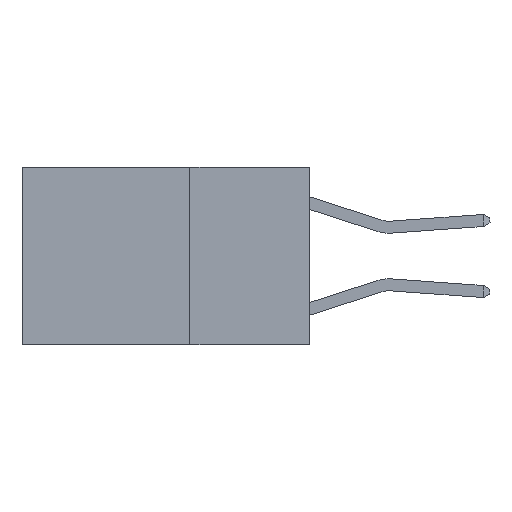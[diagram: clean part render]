
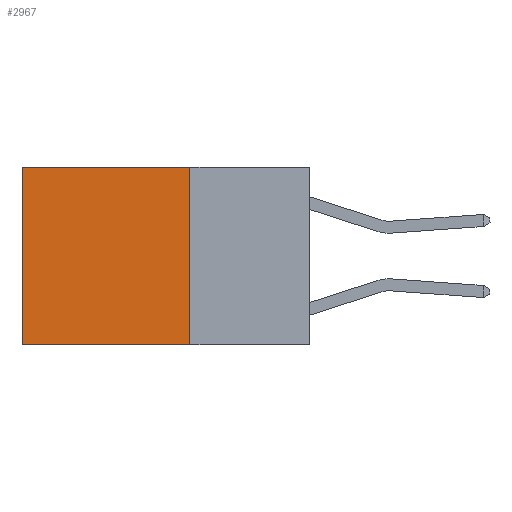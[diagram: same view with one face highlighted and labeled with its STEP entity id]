
A CAD part, left-side view. The second image highlights one B-rep face of the part: STEP entity #2967.
In plain terms, the highlighted planar face has unit normal (-1, 0, 0).
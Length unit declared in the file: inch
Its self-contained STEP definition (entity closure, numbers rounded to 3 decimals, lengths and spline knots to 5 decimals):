
#13 = EDGE_LOOP ( 'NONE', ( #6144, #16299, #10624, #16169 ) ) ;
#386 = DIRECTION ( 'NONE',  ( 0., 0., -1. ) ) ;
#877 = VECTOR ( 'NONE', #18051, 39.37008 ) ;
#1320 = VERTEX_POINT ( 'NONE', #2333 ) ;
#1862 = CARTESIAN_POINT ( 'NONE',  ( 0.2625, 0.6, 0. ) ) ;
#2333 = CARTESIAN_POINT ( 'NONE',  ( 0.2625, 0.6, -0.37 ) ) ;
#2347 = LINE ( 'NONE', #3435, #2872 ) ;
#2629 = PLANE ( 'NONE',  #9972 ) ;
#2872 = VECTOR ( 'NONE', #386, 39.37008 ) ;
#2967 = ADVANCED_FACE ( 'NONE', ( #16172 ), #2629, .F. ) ;
#3435 = CARTESIAN_POINT ( 'NONE',  ( 0.2625, 0.25, 0. ) ) ;
#3938 = CARTESIAN_POINT ( 'NONE',  ( 0.2625, 0.25, 0. ) ) ;
#4616 = CARTESIAN_POINT ( 'NONE',  ( 0.2625, 0.25, 0. ) ) ;
#4956 = EDGE_CURVE ( 'NONE', #8436, #1320, #16092, .T. ) ;
#6003 = LINE ( 'NONE', #15457, #19912 ) ;
#6144 = ORIENTED_EDGE ( 'NONE', *, *, #4956, .T. ) ;
#7473 = CARTESIAN_POINT ( 'NONE',  ( 0.2625, 0.25, -0.37 ) ) ;
#8436 = VERTEX_POINT ( 'NONE', #1862 ) ;
#8684 = DIRECTION ( 'NONE',  ( 0., 1., 0. ) ) ;
#9086 = DIRECTION ( 'NONE',  ( 0., 1., 0. ) ) ;
#9587 = CARTESIAN_POINT ( 'NONE',  ( 0.2625, 0.6, 0. ) ) ;
#9831 = LINE ( 'NONE', #20088, #16014 ) ;
#9972 = AXIS2_PLACEMENT_3D ( 'NONE', #3938, #17127, #12805 ) ;
#10485 = EDGE_CURVE ( 'NONE', #18969, #8436, #6003, .T. ) ;
#10624 = ORIENTED_EDGE ( 'NONE', *, *, #11504, .F. ) ;
#11504 = EDGE_CURVE ( 'NONE', #18969, #17571, #2347, .T. ) ;
#12805 = DIRECTION ( 'NONE',  ( 0., 0., -1. ) ) ;
#15457 = CARTESIAN_POINT ( 'NONE',  ( 0.2625, 0.25, 0. ) ) ;
#16014 = VECTOR ( 'NONE', #8684, 39.37008 ) ;
#16092 = LINE ( 'NONE', #9587, #877 ) ;
#16169 = ORIENTED_EDGE ( 'NONE', *, *, #10485, .T. ) ;
#16172 = FACE_OUTER_BOUND ( 'NONE', #13, .T. ) ;
#16299 = ORIENTED_EDGE ( 'NONE', *, *, #20673, .F. ) ;
#17127 = DIRECTION ( 'NONE',  ( 1., 0., 0. ) ) ;
#17571 = VERTEX_POINT ( 'NONE', #7473 ) ;
#18051 = DIRECTION ( 'NONE',  ( 0., 0., -1. ) ) ;
#18969 = VERTEX_POINT ( 'NONE', #4616 ) ;
#19912 = VECTOR ( 'NONE', #9086, 39.37008 ) ;
#20088 = CARTESIAN_POINT ( 'NONE',  ( 0.2625, 0.25, -0.37 ) ) ;
#20673 = EDGE_CURVE ( 'NONE', #17571, #1320, #9831, .T. ) ;
